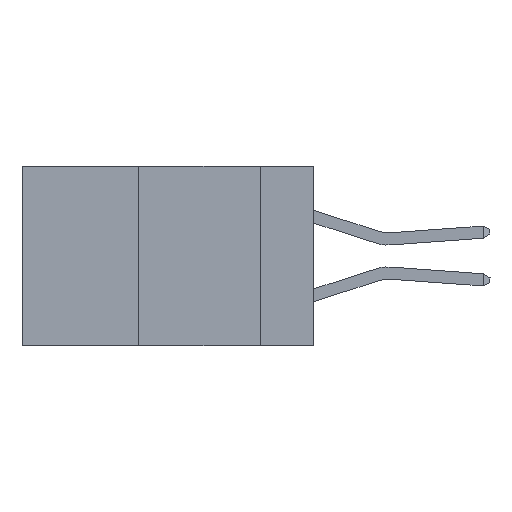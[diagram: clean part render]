
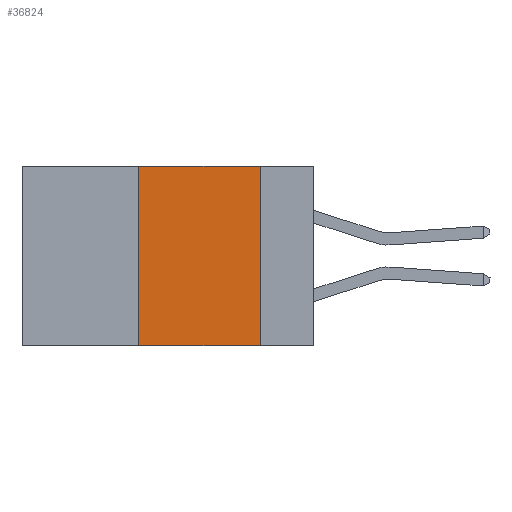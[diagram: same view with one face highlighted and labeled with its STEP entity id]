
A CAD part, left-side view. The second image highlights one B-rep face of the part: STEP entity #36824.
In plain terms, the highlighted planar face has unit normal (-1, 0, 0).
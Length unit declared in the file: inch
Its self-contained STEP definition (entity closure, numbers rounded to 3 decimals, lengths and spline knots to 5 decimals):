
#25 = CARTESIAN_POINT ( 'NONE',  ( 0., 0.6, 0. ) ) ;
#356 = CARTESIAN_POINT ( 'NONE',  ( 0., 0.11, 0. ) ) ;
#2727 = LINE ( 'NONE', #12712, #6205 ) ;
#3324 = DIRECTION ( 'NONE',  ( 0., -1., 0. ) ) ;
#5874 = VERTEX_POINT ( 'NONE', #356 ) ;
#6205 = VECTOR ( 'NONE', #3324, 39.37008 ) ;
#8938 = VERTEX_POINT ( 'NONE', #27007 ) ;
#9955 = DIRECTION ( 'NONE',  ( 0., 0., -1. ) ) ;
#12390 = FACE_OUTER_BOUND ( 'NONE', #12631, .T. ) ;
#12631 = EDGE_LOOP ( 'NONE', ( #30894, #37915, #17377, #18571 ) ) ;
#12712 = CARTESIAN_POINT ( 'NONE',  ( 0., 0.6, -0.37 ) ) ;
#12918 = PLANE ( 'NONE',  #37311 ) ;
#14108 = CARTESIAN_POINT ( 'NONE',  ( 0., 0.6, 0. ) ) ;
#17377 = ORIENTED_EDGE ( 'NONE', *, *, #33447, .F. ) ;
#18571 = ORIENTED_EDGE ( 'NONE', *, *, #33794, .T. ) ;
#20587 = DIRECTION ( 'NONE',  ( 0., -1., 0. ) ) ;
#20616 = EDGE_CURVE ( 'NONE', #27961, #5874, #22870, .T. ) ;
#22870 = LINE ( 'NONE', #14108, #28344 ) ;
#23733 = CARTESIAN_POINT ( 'NONE',  ( 0., 0.36, 0. ) ) ;
#23805 = CARTESIAN_POINT ( 'NONE',  ( 0., 0.36, 0. ) ) ;
#24625 = CARTESIAN_POINT ( 'NONE',  ( 0., 0.36, -0.37 ) ) ;
#24911 = VERTEX_POINT ( 'NONE', #24625 ) ;
#25047 = VECTOR ( 'NONE', #34656, 39.37008 ) ;
#26595 = DIRECTION ( 'NONE',  ( 0., 0., 1. ) ) ;
#26614 = EDGE_CURVE ( 'NONE', #5874, #8938, #33563, .T. ) ;
#27007 = CARTESIAN_POINT ( 'NONE',  ( 0., 0.11, -0.37 ) ) ;
#27961 = VERTEX_POINT ( 'NONE', #23733 ) ;
#28344 = VECTOR ( 'NONE', #20587, 39.37008 ) ;
#30894 = ORIENTED_EDGE ( 'NONE', *, *, #26614, .F. ) ;
#31312 = VECTOR ( 'NONE', #26595, 39.37008 ) ;
#33447 = EDGE_CURVE ( 'NONE', #24911, #27961, #40382, .T. ) ;
#33563 = LINE ( 'NONE', #38053, #25047 ) ;
#33794 = EDGE_CURVE ( 'NONE', #24911, #8938, #2727, .T. ) ;
#34656 = DIRECTION ( 'NONE',  ( 0., 0., -1. ) ) ;
#36824 = ADVANCED_FACE ( 'NONE', ( #12390 ), #12918, .F. ) ;
#37311 = AXIS2_PLACEMENT_3D ( 'NONE', #25, #38584, #9955 ) ;
#37915 = ORIENTED_EDGE ( 'NONE', *, *, #20616, .F. ) ;
#38053 = CARTESIAN_POINT ( 'NONE',  ( 0., 0.11, 0. ) ) ;
#38584 = DIRECTION ( 'NONE',  ( 1., 0., 0. ) ) ;
#40382 = LINE ( 'NONE', #23805, #31312 ) ;
